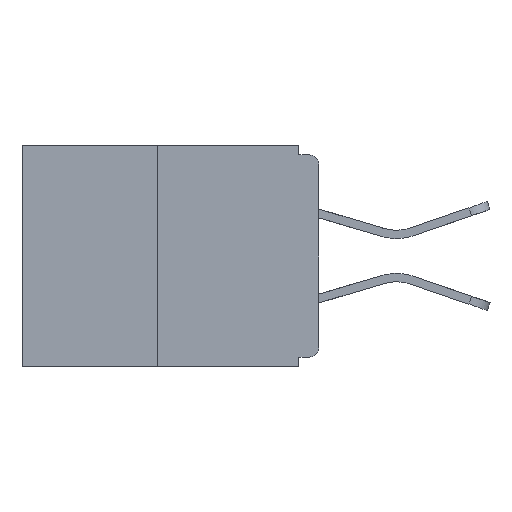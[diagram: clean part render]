
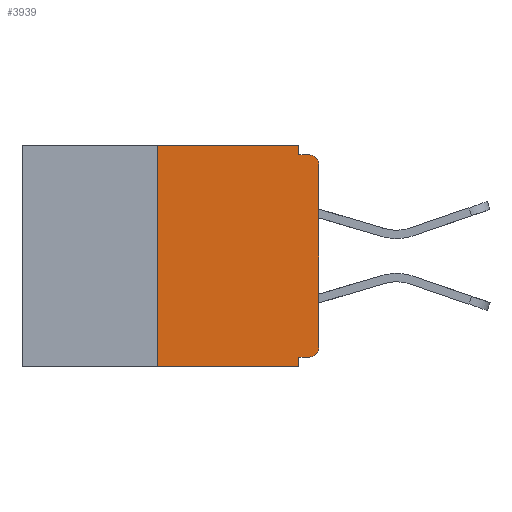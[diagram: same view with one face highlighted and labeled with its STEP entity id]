
A CAD part, left-side view. The second image highlights one B-rep face of the part: STEP entity #3939.
In plain terms, the highlighted planar face has unit normal (-1, 0, 0).
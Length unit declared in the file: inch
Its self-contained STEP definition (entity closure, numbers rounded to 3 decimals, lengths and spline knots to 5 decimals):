
#70 = CARTESIAN_POINT ( 'NONE',  ( 0., 0., -0.015 ) ) ;
#144 = VERTEX_POINT ( 'NONE', #12333 ) ;
#244 = CARTESIAN_POINT ( 'NONE',  ( 0., 0.015, -0.03 ) ) ;
#430 = LINE ( 'NONE', #1974, #3076 ) ;
#930 = EDGE_CURVE ( 'NONE', #4265, #11441, #1872, .T. ) ;
#1019 = LINE ( 'NONE', #11747, #10092 ) ;
#1189 = ORIENTED_EDGE ( 'NONE', *, *, #5057, .F. ) ;
#1329 = VECTOR ( 'NONE', #10432, 39.37008 ) ;
#1362 = VECTOR ( 'NONE', #15840, 39.37008 ) ;
#1385 = EDGE_CURVE ( 'NONE', #4001, #11011, #430, .T. ) ;
#1676 = CARTESIAN_POINT ( 'NONE',  ( 0., 0., -0.313 ) ) ;
#1714 = VERTEX_POINT ( 'NONE', #3568 ) ;
#1872 = CIRCLE ( 'NONE', #13962, 0.015 ) ;
#1974 = CARTESIAN_POINT ( 'NONE',  ( 0., 0.46, -0.343 ) ) ;
#2047 = ORIENTED_EDGE ( 'NONE', *, *, #8138, .F. ) ;
#2314 = ORIENTED_EDGE ( 'NONE', *, *, #2793, .T. ) ;
#2743 = LINE ( 'NONE', #15132, #9768 ) ;
#2793 = EDGE_CURVE ( 'NONE', #11441, #9589, #5179, .T. ) ;
#2917 = FACE_OUTER_BOUND ( 'NONE', #15717, .T. ) ;
#2940 = CARTESIAN_POINT ( 'NONE',  ( 0., 0.031, -0.328 ) ) ;
#3076 = VECTOR ( 'NONE', #9493, 39.37008 ) ;
#3568 = CARTESIAN_POINT ( 'NONE',  ( 0., 0.25, 0. ) ) ;
#3939 = ADVANCED_FACE ( 'NONE', ( #2917 ), #8965, .F. ) ;
#4001 = VERTEX_POINT ( 'NONE', #16348 ) ;
#4237 = CARTESIAN_POINT ( 'NONE',  ( 0., 0.25, 0. ) ) ;
#4265 = VERTEX_POINT ( 'NONE', #5479 ) ;
#4430 = DIRECTION ( 'NONE',  ( 0., 0., -1. ) ) ;
#4824 = VERTEX_POINT ( 'NONE', #2940 ) ;
#4927 = DIRECTION ( 'NONE',  ( 0., 0., -1. ) ) ;
#5057 = EDGE_CURVE ( 'NONE', #4001, #1714, #9710, .T. ) ;
#5077 = ORIENTED_EDGE ( 'NONE', *, *, #12527, .F. ) ;
#5179 = LINE ( 'NONE', #13111, #1329 ) ;
#5403 = ORIENTED_EDGE ( 'NONE', *, *, #10558, .F. ) ;
#5408 = ORIENTED_EDGE ( 'NONE', *, *, #9012, .F. ) ;
#5479 = CARTESIAN_POINT ( 'NONE',  ( 0., 0.015, -0.328 ) ) ;
#5709 = EDGE_CURVE ( 'NONE', #9589, #15553, #6089, .T. ) ;
#6089 = CIRCLE ( 'NONE', #13518, 0.015 ) ;
#6296 = CARTESIAN_POINT ( 'NONE',  ( 0., 0.015, -0.015 ) ) ;
#6615 = DIRECTION ( 'NONE',  ( -1., 0., 0. ) ) ;
#6742 = CARTESIAN_POINT ( 'NONE',  ( 0., 0.031, 0. ) ) ;
#6802 = LINE ( 'NONE', #6742, #10233 ) ;
#7218 = LINE ( 'NONE', #7559, #1362 ) ;
#7559 = CARTESIAN_POINT ( 'NONE',  ( 0., 0.46, 0. ) ) ;
#7992 = ORIENTED_EDGE ( 'NONE', *, *, #5709, .T. ) ;
#8138 = EDGE_CURVE ( 'NONE', #144, #9909, #6802, .T. ) ;
#8183 = AXIS2_PLACEMENT_3D ( 'NONE', #15362, #16486, #11518 ) ;
#8419 = DIRECTION ( 'NONE',  ( -1., 0., 0. ) ) ;
#8965 = PLANE ( 'NONE',  #8183 ) ;
#9012 = EDGE_CURVE ( 'NONE', #1714, #144, #7218, .T. ) ;
#9213 = DIRECTION ( 'NONE',  ( 0., 0., 1. ) ) ;
#9413 = DIRECTION ( 'NONE',  ( 0., 0., -1. ) ) ;
#9493 = DIRECTION ( 'NONE',  ( 0., -1., 0. ) ) ;
#9589 = VERTEX_POINT ( 'NONE', #15069 ) ;
#9691 = CARTESIAN_POINT ( 'NONE',  ( 0., 0.015, -0.313 ) ) ;
#9710 = LINE ( 'NONE', #4237, #14992 ) ;
#9768 = VECTOR ( 'NONE', #4430, 39.37008 ) ;
#9909 = VERTEX_POINT ( 'NONE', #16109 ) ;
#10092 = VECTOR ( 'NONE', #13053, 39.37008 ) ;
#10233 = VECTOR ( 'NONE', #11954, 39.37008 ) ;
#10432 = DIRECTION ( 'NONE',  ( 0., 0., 1. ) ) ;
#10548 = DIRECTION ( 'NONE',  ( 0., -1., 0. ) ) ;
#10558 = EDGE_CURVE ( 'NONE', #9909, #15553, #10594, .T. ) ;
#10594 = LINE ( 'NONE', #70, #16249 ) ;
#11011 = VERTEX_POINT ( 'NONE', #12639 ) ;
#11441 = VERTEX_POINT ( 'NONE', #1676 ) ;
#11518 = DIRECTION ( 'NONE',  ( 0., 0., -1. ) ) ;
#11747 = CARTESIAN_POINT ( 'NONE',  ( 0., 0., -0.328 ) ) ;
#11954 = DIRECTION ( 'NONE',  ( 0., 0., -1. ) ) ;
#12224 = ORIENTED_EDGE ( 'NONE', *, *, #1385, .T. ) ;
#12333 = CARTESIAN_POINT ( 'NONE',  ( 0., 0.031, 0. ) ) ;
#12527 = EDGE_CURVE ( 'NONE', #4265, #4824, #1019, .T. ) ;
#12639 = CARTESIAN_POINT ( 'NONE',  ( 0., 0.031, -0.343 ) ) ;
#13053 = DIRECTION ( 'NONE',  ( 0., 1., 0. ) ) ;
#13111 = CARTESIAN_POINT ( 'NONE',  ( 0., 0., 0. ) ) ;
#13518 = AXIS2_PLACEMENT_3D ( 'NONE', #244, #6615, #9413 ) ;
#13962 = AXIS2_PLACEMENT_3D ( 'NONE', #9691, #8419, #4927 ) ;
#14334 = ORIENTED_EDGE ( 'NONE', *, *, #15921, .F. ) ;
#14992 = VECTOR ( 'NONE', #9213, 39.37008 ) ;
#15069 = CARTESIAN_POINT ( 'NONE',  ( 0., 0., -0.03 ) ) ;
#15132 = CARTESIAN_POINT ( 'NONE',  ( 0., 0.031, -0.343 ) ) ;
#15362 = CARTESIAN_POINT ( 'NONE',  ( 0., 0.46, 0. ) ) ;
#15553 = VERTEX_POINT ( 'NONE', #6296 ) ;
#15717 = EDGE_LOOP ( 'NONE', ( #5408, #1189, #12224, #14334, #5077, #16009, #2314, #7992, #5403, #2047 ) ) ;
#15840 = DIRECTION ( 'NONE',  ( 0., -1., 0. ) ) ;
#15921 = EDGE_CURVE ( 'NONE', #4824, #11011, #2743, .T. ) ;
#16009 = ORIENTED_EDGE ( 'NONE', *, *, #930, .T. ) ;
#16109 = CARTESIAN_POINT ( 'NONE',  ( 0., 0.031, -0.015 ) ) ;
#16249 = VECTOR ( 'NONE', #10548, 39.37008 ) ;
#16348 = CARTESIAN_POINT ( 'NONE',  ( 0., 0.25, -0.343 ) ) ;
#16486 = DIRECTION ( 'NONE',  ( 1., 0., 0. ) ) ;
